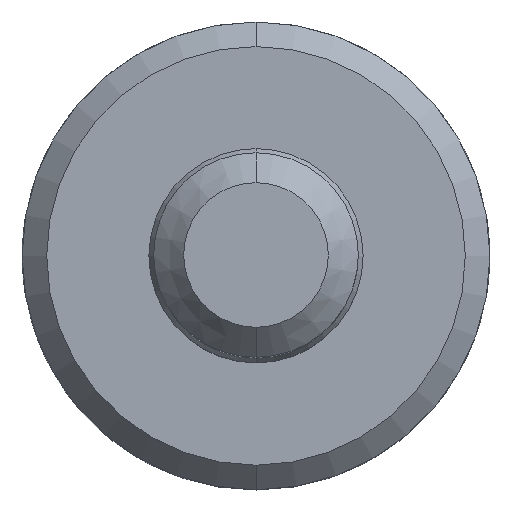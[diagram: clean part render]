
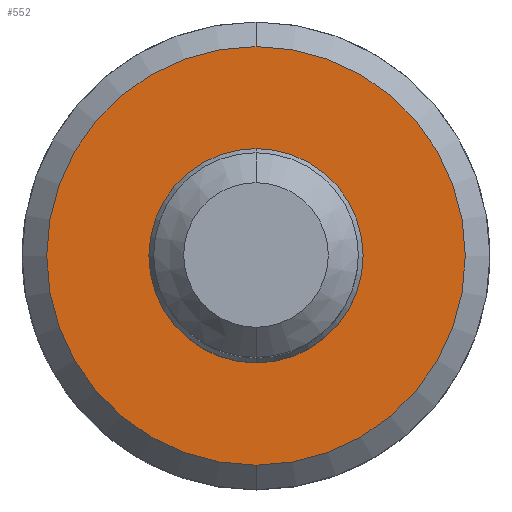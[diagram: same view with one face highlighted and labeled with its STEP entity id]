
A CAD part, top view. The second image highlights one B-rep face of the part: STEP entity #552.
In plain terms, the highlighted planar face has unit normal (0, 0, 1).
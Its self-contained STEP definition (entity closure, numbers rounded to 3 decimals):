
#37 = ORIENTED_EDGE ( 'NONE', *, *, #544, .F. ) ;
#74 = DIRECTION ( 'NONE',  ( 0., 1., 0. ) ) ;
#76 = DIRECTION ( 'NONE',  ( 0., 0., -1. ) ) ;
#78 = CARTESIAN_POINT ( 'NONE',  ( 0., 0., -13.411 ) ) ;
#149 = VERTEX_POINT ( 'NONE', #619 ) ;
#174 = AXIS2_PLACEMENT_3D ( 'NONE', #181, #451, #449 ) ;
#176 = DIRECTION ( 'NONE',  ( 0., -1., 0. ) ) ;
#177 = DIRECTION ( 'NONE',  ( 0., 0., 1. ) ) ;
#180 = CARTESIAN_POINT ( 'NONE',  ( 0., 0., -13.411 ) ) ;
#181 = CARTESIAN_POINT ( 'NONE',  ( 0., 2.832, -13.411 ) ) ;
#235 = CARTESIAN_POINT ( 'NONE',  ( 0., 5.534, -13.411 ) ) ;
#236 = CIRCLE ( 'NONE', #452, 2.832 ) ;
#246 = VERTEX_POINT ( 'NONE', #235 ) ;
#247 = AXIS2_PLACEMENT_3D ( 'NONE', #495, #494, #491 ) ;
#260 = AXIS2_PLACEMENT_3D ( 'NONE', #485, #484, #482 ) ;
#298 = CARTESIAN_POINT ( 'NONE',  ( 0., 2.832, -13.411 ) ) ;
#307 = CARTESIAN_POINT ( 'NONE',  ( 0., -2.832, -13.411 ) ) ;
#315 = CIRCLE ( 'NONE', #247, 5.534 ) ;
#341 = EDGE_LOOP ( 'NONE', ( #650, #37 ) ) ;
#363 = ORIENTED_EDGE ( 'NONE', *, *, #463, .F. ) ;
#404 = FACE_OUTER_BOUND ( 'NONE', #341, .T. ) ;
#418 = CIRCLE ( 'NONE', #441, 5.534 ) ;
#441 = AXIS2_PLACEMENT_3D ( 'NONE', #78, #76, #74 ) ;
#449 = DIRECTION ( 'NONE',  ( 0., 1., 0. ) ) ;
#451 = DIRECTION ( 'NONE',  ( 0., 0., -1. ) ) ;
#452 = AXIS2_PLACEMENT_3D ( 'NONE', #180, #177, #176 ) ;
#463 = EDGE_CURVE ( 'NONE', #631, #647, #236, .T. ) ;
#468 = PLANE ( 'NONE',  #174 ) ;
#478 = EDGE_CURVE ( 'NONE', #246, #149, #418, .T. ) ;
#482 = DIRECTION ( 'NONE',  ( 0., -1., 0. ) ) ;
#484 = DIRECTION ( 'NONE',  ( 0., 0., 1. ) ) ;
#485 = CARTESIAN_POINT ( 'NONE',  ( 0., 0., -13.411 ) ) ;
#491 = DIRECTION ( 'NONE',  ( 0., 1., 0. ) ) ;
#494 = DIRECTION ( 'NONE',  ( 0., 0., -1. ) ) ;
#495 = CARTESIAN_POINT ( 'NONE',  ( 0., 0., -13.411 ) ) ;
#544 = EDGE_CURVE ( 'NONE', #149, #246, #315, .T. ) ;
#545 = EDGE_CURVE ( 'NONE', #647, #631, #641, .T. ) ;
#552 = ADVANCED_FACE ( 'NONE', ( #404, #636 ), #468, .F. ) ;
#556 = EDGE_LOOP ( 'NONE', ( #363, #613 ) ) ;
#613 = ORIENTED_EDGE ( 'NONE', *, *, #545, .F. ) ;
#619 = CARTESIAN_POINT ( 'NONE',  ( 0., -5.534, -13.411 ) ) ;
#631 = VERTEX_POINT ( 'NONE', #307 ) ;
#636 = FACE_BOUND ( 'NONE', #556, .T. ) ;
#641 = CIRCLE ( 'NONE', #260, 2.832 ) ;
#647 = VERTEX_POINT ( 'NONE', #298 ) ;
#650 = ORIENTED_EDGE ( 'NONE', *, *, #478, .F. ) ;
